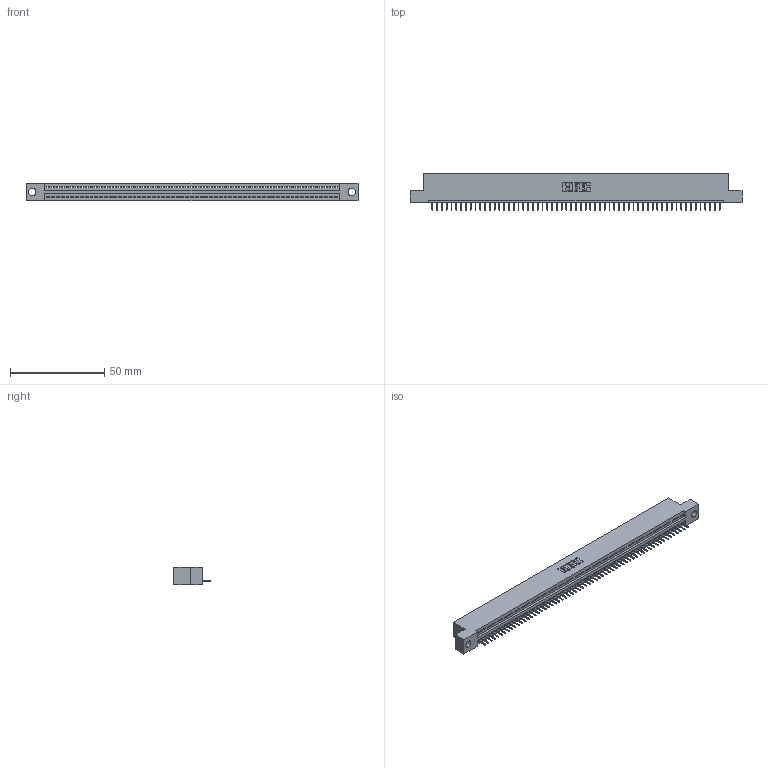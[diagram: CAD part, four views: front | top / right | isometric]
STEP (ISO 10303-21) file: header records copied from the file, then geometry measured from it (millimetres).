
FILE_DESCRIPTION (( 'STEP AP203' ), '1' );
FILE_NAME ('345-061-524-104.STEP', '2021-05-28T15:51:24', ( '' ), ( '' ), 'SwSTEP 2.0', 'SolidWorks 2020', '' );
FILE_SCHEMA (( 'CONFIG_CONTROL_DESIGN' ));
Length unit declared in the file: inch
Products named in the file (3): 345 Part_Flush Mounting Lugs - 0.156 Dia-TI; 345-292-001_345-293-124; 345-061-524-104
Assembly tree (62 placements, depth 2):
  345-061-524-104
    345 Part_Flush Mounting Lugs - 0.156 Dia-TI
    345-292-001_345-293-124  x61
Bounding box: 176.15 x 19.35 x 9.4 mm (x, y, z)
Volume: 16539.5 mm3; surface area: 21309.8 mm2
Topology: 62 solids, 62 shells, 3922 faces, 11357 edges, 7326 vertices
Faces by surface type: plane 2900, cylinder 1022
Entity records: 43845 total; most frequent: CARTESIAN_POINT 7601, ORIENTED_EDGE 7594, DIRECTION 6611, EDGE_CURVE 3797, LINE 3425, VECTOR 3425, VERTEX_POINT 2526, AXIS2_PLACEMENT_3D 1593
